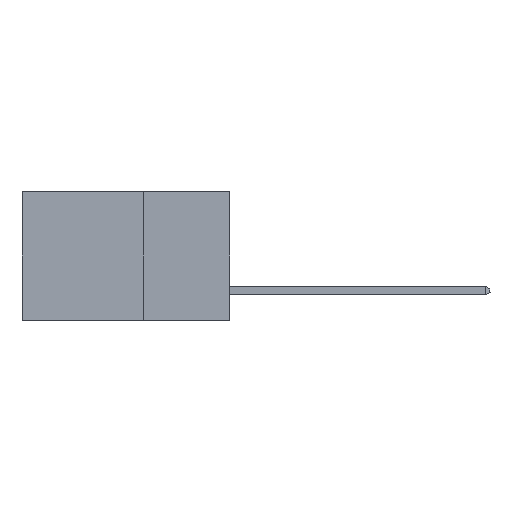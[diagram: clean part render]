
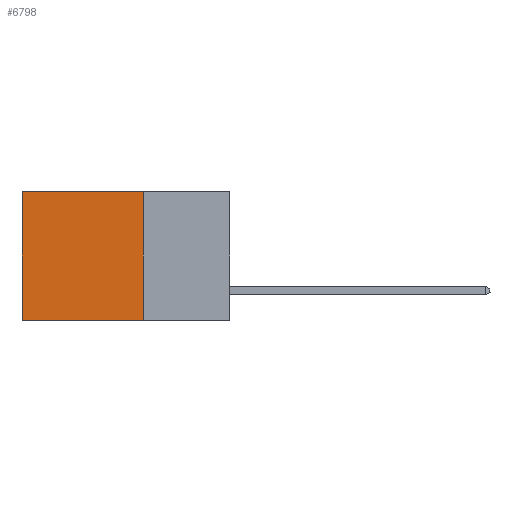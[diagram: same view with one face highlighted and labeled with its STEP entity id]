
A CAD part, left-side view. The second image highlights one B-rep face of the part: STEP entity #6798.
In plain terms, the highlighted planar face has unit normal (-1, 0, 0).
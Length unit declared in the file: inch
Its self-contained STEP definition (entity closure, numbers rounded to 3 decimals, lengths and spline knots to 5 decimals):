
#205 = ORIENTED_EDGE ( 'NONE', *, *, #4752, .T. ) ;
#356 = PLANE ( 'NONE',  #9633 ) ;
#812 = FACE_OUTER_BOUND ( 'NONE', #2685, .T. ) ;
#1729 = VERTEX_POINT ( 'NONE', #10482 ) ;
#2390 = LINE ( 'NONE', #12607, #7683 ) ;
#2685 = EDGE_LOOP ( 'NONE', ( #205, #13642, #8281, #9356 ) ) ;
#3246 = CARTESIAN_POINT ( 'NONE',  ( 0.298, 0.25, -0.37 ) ) ;
#4110 = CARTESIAN_POINT ( 'NONE',  ( 0.298, 0.25, -0.37 ) ) ;
#4162 = VERTEX_POINT ( 'NONE', #4699 ) ;
#4699 = CARTESIAN_POINT ( 'NONE',  ( 0.298, 0.6, -0.37 ) ) ;
#4752 = EDGE_CURVE ( 'NONE', #1729, #4162, #2390, .T. ) ;
#4891 = VECTOR ( 'NONE', #12932, 39.37008 ) ;
#4952 = CARTESIAN_POINT ( 'NONE',  ( 0.298, 0.25, 0. ) ) ;
#5311 = DIRECTION ( 'NONE',  ( 0., 0., -1. ) ) ;
#5544 = LINE ( 'NONE', #3246, #11142 ) ;
#5891 = DIRECTION ( 'NONE',  ( 0., 0., -1. ) ) ;
#6122 = DIRECTION ( 'NONE',  ( 0., 0., -1. ) ) ;
#6666 = CARTESIAN_POINT ( 'NONE',  ( 0.298, 0.25, 0. ) ) ;
#6798 = ADVANCED_FACE ( 'NONE', ( #812 ), #356, .F. ) ;
#7148 = EDGE_CURVE ( 'NONE', #11423, #1729, #7286, .T. ) ;
#7286 = LINE ( 'NONE', #6666, #4891 ) ;
#7531 = DIRECTION ( 'NONE',  ( 0., 1., 0. ) ) ;
#7683 = VECTOR ( 'NONE', #6122, 39.37008 ) ;
#8281 = ORIENTED_EDGE ( 'NONE', *, *, #11766, .F. ) ;
#8687 = CARTESIAN_POINT ( 'NONE',  ( 0.298, 0.25, 0. ) ) ;
#9356 = ORIENTED_EDGE ( 'NONE', *, *, #7148, .T. ) ;
#9592 = CARTESIAN_POINT ( 'NONE',  ( 0.298, 0.25, 0. ) ) ;
#9633 = AXIS2_PLACEMENT_3D ( 'NONE', #4952, #10378, #5891 ) ;
#10321 = EDGE_CURVE ( 'NONE', #12052, #4162, #5544, .T. ) ;
#10378 = DIRECTION ( 'NONE',  ( 1., 0., 0. ) ) ;
#10482 = CARTESIAN_POINT ( 'NONE',  ( 0.298, 0.6, 0. ) ) ;
#10568 = VECTOR ( 'NONE', #5311, 39.37008 ) ;
#11142 = VECTOR ( 'NONE', #7531, 39.37008 ) ;
#11423 = VERTEX_POINT ( 'NONE', #9592 ) ;
#11766 = EDGE_CURVE ( 'NONE', #11423, #12052, #12935, .T. ) ;
#12052 = VERTEX_POINT ( 'NONE', #4110 ) ;
#12607 = CARTESIAN_POINT ( 'NONE',  ( 0.298, 0.6, 0. ) ) ;
#12932 = DIRECTION ( 'NONE',  ( 0., 1., 0. ) ) ;
#12935 = LINE ( 'NONE', #8687, #10568 ) ;
#13642 = ORIENTED_EDGE ( 'NONE', *, *, #10321, .F. ) ;
